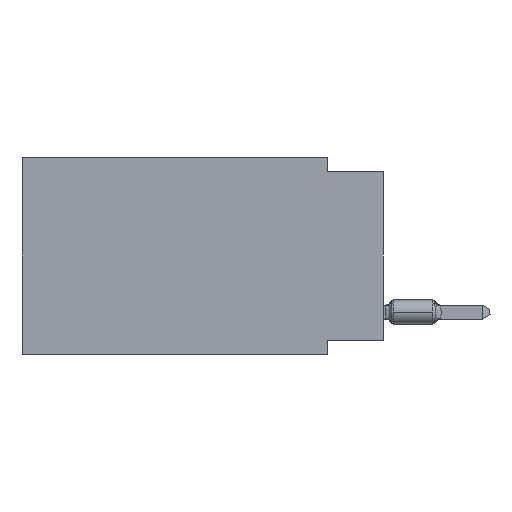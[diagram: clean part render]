
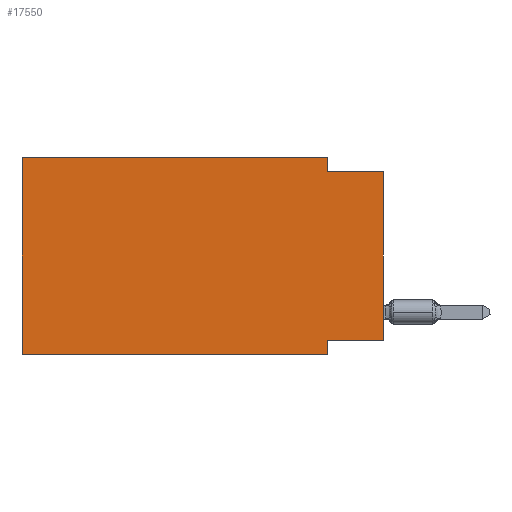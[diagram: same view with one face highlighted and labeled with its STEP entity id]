
A CAD part, left-side view. The second image highlights one B-rep face of the part: STEP entity #17550.
In plain terms, the highlighted planar face has unit normal (-1, 0, 0).
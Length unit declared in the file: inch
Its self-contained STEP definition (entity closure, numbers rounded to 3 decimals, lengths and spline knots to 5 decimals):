
#1540 = VECTOR ( 'NONE', #25148, 39.37008 ) ;
#1790 = CARTESIAN_POINT ( 'NONE',  ( 0., 0.1, -0.025 ) ) ;
#2453 = DIRECTION ( 'NONE',  ( 0., 0., -1. ) ) ;
#2462 = CARTESIAN_POINT ( 'NONE',  ( 0., 0.645, 0. ) ) ;
#3409 = EDGE_LOOP ( 'NONE', ( #26662, #30868, #22324, #29731, #4141, #10386, #17334, #27669 ) ) ;
#3413 = VECTOR ( 'NONE', #21780, 39.37008 ) ;
#4141 = ORIENTED_EDGE ( 'NONE', *, *, #16654, .F. ) ;
#4530 = VECTOR ( 'NONE', #21531, 39.37008 ) ;
#4546 = AXIS2_PLACEMENT_3D ( 'NONE', #2462, #7704, #9758 ) ;
#4588 = EDGE_CURVE ( 'NONE', #30440, #8582, #4983, .T. ) ;
#4983 = LINE ( 'NONE', #25719, #33474 ) ;
#6018 = CARTESIAN_POINT ( 'NONE',  ( 0., 0.1, -0.35 ) ) ;
#6380 = DIRECTION ( 'NONE',  ( 0., -1., 0. ) ) ;
#7704 = DIRECTION ( 'NONE',  ( 1., 0., 0. ) ) ;
#7708 = LINE ( 'NONE', #8692, #3413 ) ;
#8012 = DIRECTION ( 'NONE',  ( 0., 0., 1. ) ) ;
#8582 = VERTEX_POINT ( 'NONE', #6018 ) ;
#8692 = CARTESIAN_POINT ( 'NONE',  ( 0., 0.645, -0.35 ) ) ;
#9101 = CARTESIAN_POINT ( 'NONE',  ( 0., 0.1, 0. ) ) ;
#9758 = DIRECTION ( 'NONE',  ( 0., 0., -1. ) ) ;
#10386 = ORIENTED_EDGE ( 'NONE', *, *, #16235, .T. ) ;
#11058 = VERTEX_POINT ( 'NONE', #11828 ) ;
#11662 = LINE ( 'NONE', #29663, #22164 ) ;
#11828 = CARTESIAN_POINT ( 'NONE',  ( 0., 0.1, 0. ) ) ;
#12824 = EDGE_CURVE ( 'NONE', #12936, #18040, #11662, .T. ) ;
#12936 = VERTEX_POINT ( 'NONE', #1790 ) ;
#12950 = VECTOR ( 'NONE', #8012, 39.37008 ) ;
#13359 = VERTEX_POINT ( 'NONE', #25525 ) ;
#14563 = EDGE_CURVE ( 'NONE', #29843, #11058, #24369, .T. ) ;
#14992 = EDGE_CURVE ( 'NONE', #13359, #18040, #23840, .T. ) ;
#15359 = VECTOR ( 'NONE', #32317, 39.37008 ) ;
#16203 = DIRECTION ( 'NONE',  ( 0., -1., 0. ) ) ;
#16235 = EDGE_CURVE ( 'NONE', #29044, #8582, #7708, .T. ) ;
#16654 = EDGE_CURVE ( 'NONE', #29044, #29843, #20044, .T. ) ;
#17247 = VECTOR ( 'NONE', #16203, 39.37008 ) ;
#17334 = ORIENTED_EDGE ( 'NONE', *, *, #4588, .F. ) ;
#17550 = ADVANCED_FACE ( 'NONE', ( #20470 ), #30994, .F. ) ;
#18040 = VERTEX_POINT ( 'NONE', #25833 ) ;
#18372 = EDGE_CURVE ( 'NONE', #13359, #30440, #33304, .T. ) ;
#18755 = CARTESIAN_POINT ( 'NONE',  ( 0., 0.645, 0. ) ) ;
#20044 = LINE ( 'NONE', #21947, #15359 ) ;
#20470 = FACE_OUTER_BOUND ( 'NONE', #3409, .T. ) ;
#21531 = DIRECTION ( 'NONE',  ( 0., 0., -1. ) ) ;
#21780 = DIRECTION ( 'NONE',  ( 0., -1., 0. ) ) ;
#21947 = CARTESIAN_POINT ( 'NONE',  ( 0., 0.645, 0. ) ) ;
#22164 = VECTOR ( 'NONE', #6380, 39.37008 ) ;
#22324 = ORIENTED_EDGE ( 'NONE', *, *, #33332, .F. ) ;
#23840 = LINE ( 'NONE', #31641, #12950 ) ;
#24369 = LINE ( 'NONE', #18755, #17247 ) ;
#25148 = DIRECTION ( 'NONE',  ( 0., 1., 0. ) ) ;
#25525 = CARTESIAN_POINT ( 'NONE',  ( 0., 0., -0.325 ) ) ;
#25719 = CARTESIAN_POINT ( 'NONE',  ( 0., 0.1, -0.35 ) ) ;
#25833 = CARTESIAN_POINT ( 'NONE',  ( 0., 0., -0.025 ) ) ;
#26662 = ORIENTED_EDGE ( 'NONE', *, *, #14992, .T. ) ;
#27669 = ORIENTED_EDGE ( 'NONE', *, *, #18372, .F. ) ;
#29044 = VERTEX_POINT ( 'NONE', #29653 ) ;
#29653 = CARTESIAN_POINT ( 'NONE',  ( 0., 0.645, -0.35 ) ) ;
#29663 = CARTESIAN_POINT ( 'NONE',  ( 0., 0., -0.025 ) ) ;
#29731 = ORIENTED_EDGE ( 'NONE', *, *, #14563, .F. ) ;
#29843 = VERTEX_POINT ( 'NONE', #30365 ) ;
#30365 = CARTESIAN_POINT ( 'NONE',  ( 0., 0.645, 0. ) ) ;
#30440 = VERTEX_POINT ( 'NONE', #31163 ) ;
#30868 = ORIENTED_EDGE ( 'NONE', *, *, #12824, .F. ) ;
#30994 = PLANE ( 'NONE',  #4546 ) ;
#31163 = CARTESIAN_POINT ( 'NONE',  ( 0., 0.1, -0.325 ) ) ;
#31641 = CARTESIAN_POINT ( 'NONE',  ( 0., 0., 0. ) ) ;
#32317 = DIRECTION ( 'NONE',  ( 0., 0., 1. ) ) ;
#32395 = LINE ( 'NONE', #9101, #4530 ) ;
#32800 = CARTESIAN_POINT ( 'NONE',  ( 0., 0., -0.325 ) ) ;
#33304 = LINE ( 'NONE', #32800, #1540 ) ;
#33332 = EDGE_CURVE ( 'NONE', #11058, #12936, #32395, .T. ) ;
#33474 = VECTOR ( 'NONE', #2453, 39.37008 ) ;
